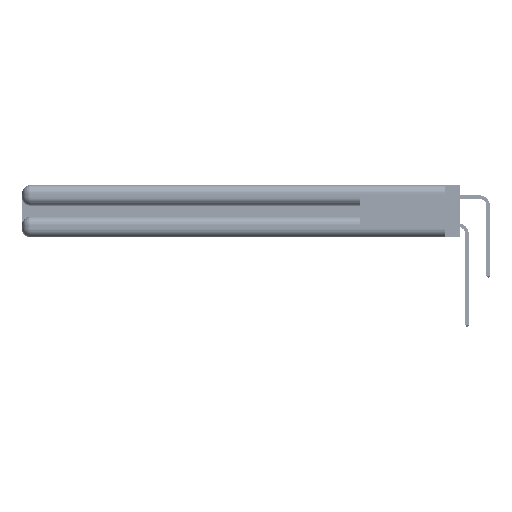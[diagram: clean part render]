
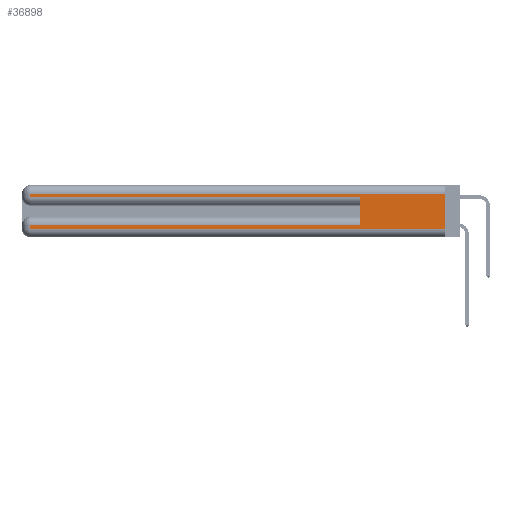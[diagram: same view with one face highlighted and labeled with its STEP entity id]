
A CAD part, left-side view. The second image highlights one B-rep face of the part: STEP entity #36898.
In plain terms, the highlighted planar face has unit normal (-1, 0, 0).
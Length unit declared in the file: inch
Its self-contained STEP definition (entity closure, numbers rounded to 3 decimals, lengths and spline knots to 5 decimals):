
#1082 = CARTESIAN_POINT ( 'NONE',  ( 0., 0., 0.06 ) ) ;
#1391 = EDGE_CURVE ( 'NONE', #45623, #10859, #54394, .T. ) ;
#1544 = ORIENTED_EDGE ( 'NONE', *, *, #29489, .T. ) ;
#4264 = CARTESIAN_POINT ( 'NONE',  ( 0., 2.94, 0.37 ) ) ;
#4619 = CARTESIAN_POINT ( 'NONE',  ( 0., 0.6, 0.085 ) ) ;
#5448 = CARTESIAN_POINT ( 'NONE',  ( 0., 0., 0.285 ) ) ;
#5533 = VECTOR ( 'NONE', #41251, 39.37008 ) ;
#6210 = LINE ( 'NONE', #4264, #19064 ) ;
#6423 = LINE ( 'NONE', #7243, #49865 ) ;
#7243 = CARTESIAN_POINT ( 'NONE',  ( 0., 0., 0.085 ) ) ;
#8959 = EDGE_CURVE ( 'NONE', #52619, #50335, #36352, .T. ) ;
#9332 = ORIENTED_EDGE ( 'NONE', *, *, #46266, .T. ) ;
#9972 = LINE ( 'NONE', #20621, #31650 ) ;
#10341 = ORIENTED_EDGE ( 'NONE', *, *, #40648, .T. ) ;
#10859 = VERTEX_POINT ( 'NONE', #25872 ) ;
#11999 = CARTESIAN_POINT ( 'NONE',  ( 0., 0., 0.37 ) ) ;
#12103 = FACE_OUTER_BOUND ( 'NONE', #39325, .T. ) ;
#12110 = EDGE_CURVE ( 'NONE', #45623, #14984, #52970, .T. ) ;
#12158 = ORIENTED_EDGE ( 'NONE', *, *, #1391, .T. ) ;
#13199 = CARTESIAN_POINT ( 'NONE',  ( 0., 0., 0.37 ) ) ;
#14132 = DIRECTION ( 'NONE',  ( 0., -1., 0. ) ) ;
#14563 = EDGE_CURVE ( 'NONE', #10859, #27446, #9972, .T. ) ;
#14984 = VERTEX_POINT ( 'NONE', #54376 ) ;
#16264 = DIRECTION ( 'NONE',  ( 0., 0., -1. ) ) ;
#17553 = DIRECTION ( 'NONE',  ( 0., 0., -1. ) ) ;
#19064 = VECTOR ( 'NONE', #38941, 39.37008 ) ;
#20621 = CARTESIAN_POINT ( 'NONE',  ( 0., 2.94, 0.37 ) ) ;
#20861 = VECTOR ( 'NONE', #22821, 39.37008 ) ;
#22121 = EDGE_CURVE ( 'NONE', #52619, #41201, #6423, .T. ) ;
#22821 = DIRECTION ( 'NONE',  ( 0., -1., 0. ) ) ;
#23338 = CARTESIAN_POINT ( 'NONE',  ( 0., 2.94, 0.085 ) ) ;
#23681 = DIRECTION ( 'NONE',  ( 0., 0., 1. ) ) ;
#23765 = VECTOR ( 'NONE', #14132, 39.37008 ) ;
#23929 = CARTESIAN_POINT ( 'NONE',  ( 0., 2.94, 0.285 ) ) ;
#24772 = VECTOR ( 'NONE', #23681, 39.37008 ) ;
#24853 = ORIENTED_EDGE ( 'NONE', *, *, #22121, .T. ) ;
#25872 = CARTESIAN_POINT ( 'NONE',  ( 0., 2.94, 0.31 ) ) ;
#26501 = CARTESIAN_POINT ( 'NONE',  ( 0., 2.94, 0.06 ) ) ;
#27446 = VERTEX_POINT ( 'NONE', #23929 ) ;
#28454 = VECTOR ( 'NONE', #33772, 39.37008 ) ;
#29489 = EDGE_CURVE ( 'NONE', #41201, #33798, #6210, .T. ) ;
#31650 = VECTOR ( 'NONE', #16264, 39.37008 ) ;
#33535 = DIRECTION ( 'NONE',  ( 0., 1., 0. ) ) ;
#33753 = LINE ( 'NONE', #1082, #20861 ) ;
#33772 = DIRECTION ( 'NONE',  ( 0., 0., -1. ) ) ;
#33798 = VERTEX_POINT ( 'NONE', #26501 ) ;
#35407 = AXIS2_PLACEMENT_3D ( 'NONE', #13199, #43570, #17553 ) ;
#36352 = LINE ( 'NONE', #41016, #24772 ) ;
#36715 = LINE ( 'NONE', #5448, #23765 ) ;
#36898 = ADVANCED_FACE ( 'NONE', ( #12103 ), #39204, .F. ) ;
#38941 = DIRECTION ( 'NONE',  ( 0., 0., -1. ) ) ;
#39204 = PLANE ( 'NONE',  #35407 ) ;
#39325 = EDGE_LOOP ( 'NONE', ( #39565, #12158, #49692, #9332, #55817, #24853, #1544, #10341 ) ) ;
#39565 = ORIENTED_EDGE ( 'NONE', *, *, #12110, .F. ) ;
#40648 = EDGE_CURVE ( 'NONE', #33798, #14984, #33753, .T. ) ;
#41016 = CARTESIAN_POINT ( 'NONE',  ( 0., 0.6, 0.145 ) ) ;
#41201 = VERTEX_POINT ( 'NONE', #23338 ) ;
#41251 = DIRECTION ( 'NONE',  ( 0., 1., 0. ) ) ;
#43570 = DIRECTION ( 'NONE',  ( 1., 0., 0. ) ) ;
#44948 = CARTESIAN_POINT ( 'NONE',  ( 0., 0., 0.31 ) ) ;
#45623 = VERTEX_POINT ( 'NONE', #44948 ) ;
#46266 = EDGE_CURVE ( 'NONE', #27446, #50335, #36715, .T. ) ;
#49692 = ORIENTED_EDGE ( 'NONE', *, *, #14563, .T. ) ;
#49865 = VECTOR ( 'NONE', #33535, 39.37008 ) ;
#49966 = CARTESIAN_POINT ( 'NONE',  ( 0., 0., 0.31 ) ) ;
#50335 = VERTEX_POINT ( 'NONE', #51790 ) ;
#51790 = CARTESIAN_POINT ( 'NONE',  ( 0., 0.6, 0.285 ) ) ;
#52619 = VERTEX_POINT ( 'NONE', #4619 ) ;
#52970 = LINE ( 'NONE', #11999, #28454 ) ;
#54376 = CARTESIAN_POINT ( 'NONE',  ( 0., 0., 0.06 ) ) ;
#54394 = LINE ( 'NONE', #49966, #5533 ) ;
#55817 = ORIENTED_EDGE ( 'NONE', *, *, #8959, .F. ) ;
